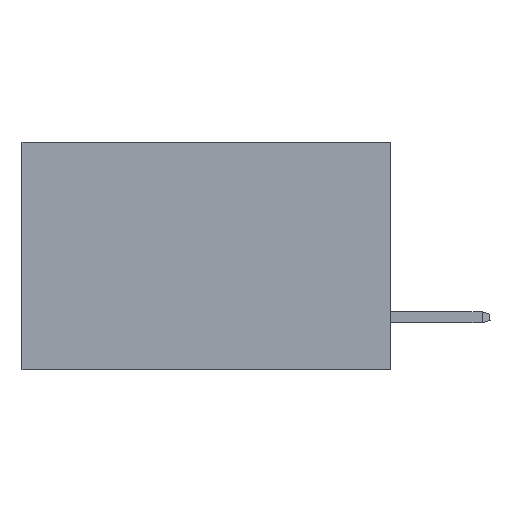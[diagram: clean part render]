
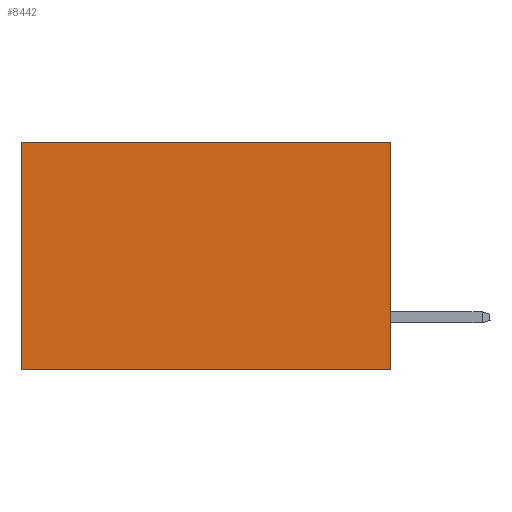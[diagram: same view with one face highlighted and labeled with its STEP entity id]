
A CAD part, left-side view. The second image highlights one B-rep face of the part: STEP entity #8442.
In plain terms, the highlighted planar face has unit normal (-1, 0, 0).
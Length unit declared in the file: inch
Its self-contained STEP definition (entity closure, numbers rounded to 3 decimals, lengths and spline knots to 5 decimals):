
#84 = CARTESIAN_POINT ( 'NONE',  ( 0.2875, 0.6, 0. ) ) ;
#1814 = VERTEX_POINT ( 'NONE', #16007 ) ;
#1828 = CARTESIAN_POINT ( 'NONE',  ( 0.2875, 0., -0.37 ) ) ;
#1889 = DIRECTION ( 'NONE',  ( 0., 1., 0. ) ) ;
#2251 = EDGE_CURVE ( 'NONE', #11387, #14015, #16391, .T. ) ;
#2343 = DIRECTION ( 'NONE',  ( 0., 1., 0. ) ) ;
#2559 = PLANE ( 'NONE',  #14282 ) ;
#2651 = CARTESIAN_POINT ( 'NONE',  ( 0.2875, 0.6, -0.37 ) ) ;
#2927 = EDGE_CURVE ( 'NONE', #1814, #14015, #15904, .T. ) ;
#3509 = ORIENTED_EDGE ( 'NONE', *, *, #2251, .F. ) ;
#3673 = CARTESIAN_POINT ( 'NONE',  ( 0.2875, 0., 0. ) ) ;
#4857 = EDGE_CURVE ( 'NONE', #11106, #11387, #9170, .T. ) ;
#4994 = VECTOR ( 'NONE', #17620, 39.37008 ) ;
#5040 = CARTESIAN_POINT ( 'NONE',  ( 0.2875, 0., 0. ) ) ;
#5331 = VECTOR ( 'NONE', #2343, 39.37008 ) ;
#5768 = LINE ( 'NONE', #3673, #5331 ) ;
#8237 = CARTESIAN_POINT ( 'NONE',  ( 0.2875, 0., 0. ) ) ;
#8442 = ADVANCED_FACE ( 'NONE', ( #16144 ), #2559, .F. ) ;
#9170 = LINE ( 'NONE', #17709, #16697 ) ;
#9613 = DIRECTION ( 'NONE',  ( 0., 0., -1. ) ) ;
#10122 = VECTOR ( 'NONE', #1889, 39.37008 ) ;
#10653 = ORIENTED_EDGE ( 'NONE', *, *, #4857, .F. ) ;
#11106 = VERTEX_POINT ( 'NONE', #5040 ) ;
#11387 = VERTEX_POINT ( 'NONE', #15280 ) ;
#13885 = EDGE_CURVE ( 'NONE', #11106, #1814, #5768, .T. ) ;
#14015 = VERTEX_POINT ( 'NONE', #2651 ) ;
#14064 = ORIENTED_EDGE ( 'NONE', *, *, #13885, .T. ) ;
#14282 = AXIS2_PLACEMENT_3D ( 'NONE', #8237, #17605, #9613 ) ;
#14410 = EDGE_LOOP ( 'NONE', ( #17509, #3509, #10653, #14064 ) ) ;
#15280 = CARTESIAN_POINT ( 'NONE',  ( 0.2875, 0., -0.37 ) ) ;
#15430 = DIRECTION ( 'NONE',  ( 0., 0., -1. ) ) ;
#15904 = LINE ( 'NONE', #84, #4994 ) ;
#16007 = CARTESIAN_POINT ( 'NONE',  ( 0.2875, 0.6, 0. ) ) ;
#16144 = FACE_OUTER_BOUND ( 'NONE', #14410, .T. ) ;
#16391 = LINE ( 'NONE', #1828, #10122 ) ;
#16697 = VECTOR ( 'NONE', #15430, 39.37008 ) ;
#17509 = ORIENTED_EDGE ( 'NONE', *, *, #2927, .T. ) ;
#17605 = DIRECTION ( 'NONE',  ( 1., 0., 0. ) ) ;
#17620 = DIRECTION ( 'NONE',  ( 0., 0., -1. ) ) ;
#17709 = CARTESIAN_POINT ( 'NONE',  ( 0.2875, 0., 0. ) ) ;
